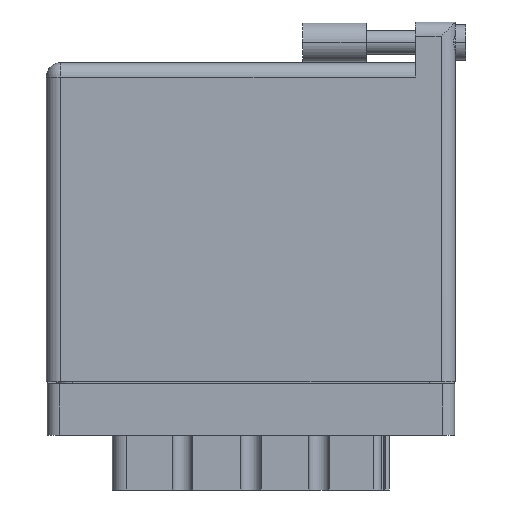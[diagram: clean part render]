
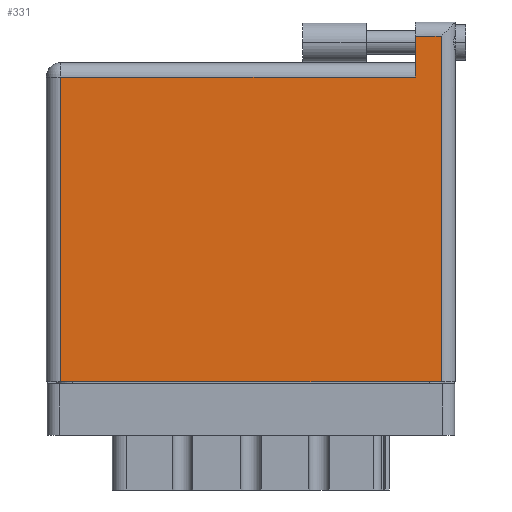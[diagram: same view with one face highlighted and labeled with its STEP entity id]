
A CAD part, front view. The second image highlights one B-rep face of the part: STEP entity #331.
In plain terms, the highlighted face is planar.
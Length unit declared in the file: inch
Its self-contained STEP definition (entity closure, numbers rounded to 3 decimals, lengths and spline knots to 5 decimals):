
#331 = ADVANCED_FACE ( 'NONE', ( #13482 ), #32282, .F. ) ;
#517 = DIRECTION ( 'NONE',  ( 1., 0., 0. ) ) ;
#520 = EDGE_CURVE ( 'NONE', #33894, #13975, #10800, .T. ) ;
#1360 = VERTEX_POINT ( 'NONE', #9434 ) ;
#1567 = AXIS2_PLACEMENT_3D ( 'NONE', #15164, #32532, #14917 ) ;
#5227 = VECTOR ( 'NONE', #517, 39.37008 ) ;
#5425 = ORIENTED_EDGE ( 'NONE', *, *, #15102, .T. ) ;
#6134 = DIRECTION ( 'NONE',  ( 0., 1., 0. ) ) ;
#6340 = CARTESIAN_POINT ( 'NONE',  ( 0., 0., 0. ) ) ;
#7891 = DIRECTION ( 'NONE',  ( -1., 0., 0. ) ) ;
#8341 = DIRECTION ( 'NONE',  ( -1., 0., 0. ) ) ;
#9202 = CARTESIAN_POINT ( 'NONE',  ( 1.811, 1.496, 0. ) ) ;
#9434 = CARTESIAN_POINT ( 'NONE',  ( 1.938, 0., 0. ) ) ;
#10800 = LINE ( 'NONE', #22311, #25028 ) ;
#13205 = ORIENTED_EDGE ( 'NONE', *, *, #28207, .T. ) ;
#13482 = FACE_OUTER_BOUND ( 'NONE', #16149, .T. ) ;
#13718 = DIRECTION ( 'NONE',  ( 0., -1., 0. ) ) ;
#13975 = VERTEX_POINT ( 'NONE', #26692 ) ;
#14296 = VECTOR ( 'NONE', #8341, 39.37008 ) ;
#14917 = DIRECTION ( 'NONE',  ( -1., 0., 0. ) ) ;
#15102 = EDGE_CURVE ( 'NONE', #25087, #36664, #27193, .T. ) ;
#15164 = CARTESIAN_POINT ( 'NONE',  ( 0., 1.566, 0. ) ) ;
#15181 = LINE ( 'NONE', #22541, #14296 ) ;
#15938 = VECTOR ( 'NONE', #17842, 39.37008 ) ;
#16149 = EDGE_LOOP ( 'NONE', ( #30546, #33898, #5425, #32086, #13205, #16932 ) ) ;
#16932 = ORIENTED_EDGE ( 'NONE', *, *, #520, .T. ) ;
#17842 = DIRECTION ( 'NONE',  ( 0., -1., 0. ) ) ;
#18980 = CARTESIAN_POINT ( 'NONE',  ( 0.07, 1.496, 0. ) ) ;
#21441 = EDGE_CURVE ( 'NONE', #36664, #26588, #21731, .T. ) ;
#21731 = LINE ( 'NONE', #34575, #15938 ) ;
#22311 = CARTESIAN_POINT ( 'NONE',  ( 0.07, 0., 0. ) ) ;
#22541 = CARTESIAN_POINT ( 'NONE',  ( 0., 1.496, 0. ) ) ;
#23548 = CARTESIAN_POINT ( 'NONE',  ( 1.938, 1.766, 0. ) ) ;
#23943 = CARTESIAN_POINT ( 'NONE',  ( 1.938, 1.696, 0. ) ) ;
#25028 = VECTOR ( 'NONE', #13718, 39.37008 ) ;
#25087 = VERTEX_POINT ( 'NONE', #23943 ) ;
#26588 = VERTEX_POINT ( 'NONE', #9202 ) ;
#26692 = CARTESIAN_POINT ( 'NONE',  ( 0.07, 0., 0. ) ) ;
#26879 = VECTOR ( 'NONE', #6134, 39.37008 ) ;
#27193 = LINE ( 'NONE', #30741, #35686 ) ;
#28207 = EDGE_CURVE ( 'NONE', #26588, #33894, #15181, .T. ) ;
#29247 = CARTESIAN_POINT ( 'NONE',  ( 1.811, 1.696, 0. ) ) ;
#30546 = ORIENTED_EDGE ( 'NONE', *, *, #31301, .T. ) ;
#30741 = CARTESIAN_POINT ( 'NONE',  ( 0., 1.696, 0. ) ) ;
#31301 = EDGE_CURVE ( 'NONE', #13975, #1360, #32047, .T. ) ;
#32047 = LINE ( 'NONE', #6340, #5227 ) ;
#32086 = ORIENTED_EDGE ( 'NONE', *, *, #21441, .T. ) ;
#32282 = PLANE ( 'NONE',  #1567 ) ;
#32532 = DIRECTION ( 'NONE',  ( 0., 0., -1. ) ) ;
#33894 = VERTEX_POINT ( 'NONE', #18980 ) ;
#33898 = ORIENTED_EDGE ( 'NONE', *, *, #34280, .T. ) ;
#34280 = EDGE_CURVE ( 'NONE', #1360, #25087, #34901, .T. ) ;
#34575 = CARTESIAN_POINT ( 'NONE',  ( 1.811, 1.766, 0. ) ) ;
#34901 = LINE ( 'NONE', #23548, #26879 ) ;
#35686 = VECTOR ( 'NONE', #7891, 39.37008 ) ;
#36664 = VERTEX_POINT ( 'NONE', #29247 ) ;
